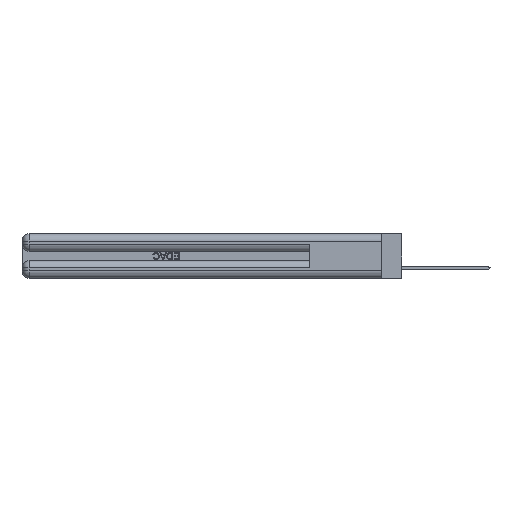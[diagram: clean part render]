
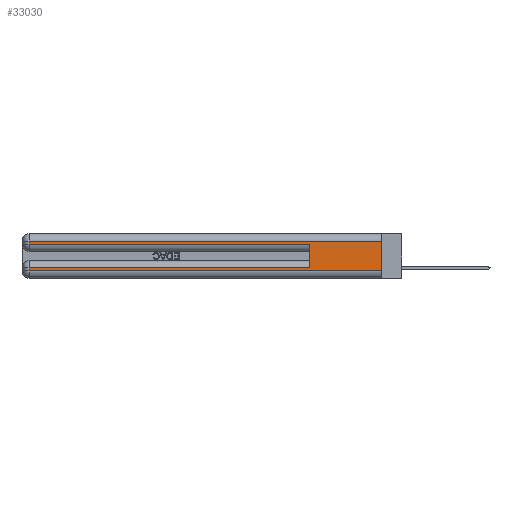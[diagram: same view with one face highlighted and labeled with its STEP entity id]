
A CAD part, left-side view. The second image highlights one B-rep face of the part: STEP entity #33030.
In plain terms, the highlighted planar face has unit normal (-1, 0, 0).
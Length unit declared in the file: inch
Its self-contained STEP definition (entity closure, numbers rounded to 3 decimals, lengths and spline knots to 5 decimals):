
#317 = VECTOR ( 'NONE', #15573, 39.37008 ) ;
#2219 = VECTOR ( 'NONE', #38193, 39.37008 ) ;
#2583 = CARTESIAN_POINT ( 'NONE',  ( 0., 0., 0.285 ) ) ;
#4704 = CARTESIAN_POINT ( 'NONE',  ( 0., 2.94, 0.31 ) ) ;
#5148 = ORIENTED_EDGE ( 'NONE', *, *, #36688, .F. ) ;
#5381 = ORIENTED_EDGE ( 'NONE', *, *, #43625, .T. ) ;
#7303 = AXIS2_PLACEMENT_3D ( 'NONE', #7928, #7403, #38817 ) ;
#7403 = DIRECTION ( 'NONE',  ( 1., 0., 0. ) ) ;
#7928 = CARTESIAN_POINT ( 'NONE',  ( 0., 0., 0.37 ) ) ;
#8430 = CARTESIAN_POINT ( 'NONE',  ( 0., 2.94, 0.06 ) ) ;
#8890 = VERTEX_POINT ( 'NONE', #9918 ) ;
#8986 = VECTOR ( 'NONE', #20823, 39.37008 ) ;
#9659 = CARTESIAN_POINT ( 'NONE',  ( 0., 0.6, 0.085 ) ) ;
#9918 = CARTESIAN_POINT ( 'NONE',  ( 0., 0., 0.31 ) ) ;
#10131 = EDGE_CURVE ( 'NONE', #13075, #24153, #19626, .T. ) ;
#10475 = DIRECTION ( 'NONE',  ( 0., 1., 0. ) ) ;
#11137 = PLANE ( 'NONE',  #7303 ) ;
#11789 = EDGE_LOOP ( 'NONE', ( #5148, #37324, #28812, #5381, #29724, #42980, #38608, #28479 ) ) ;
#11887 = EDGE_CURVE ( 'NONE', #49814, #44745, #32303, .T. ) ;
#12212 = CARTESIAN_POINT ( 'NONE',  ( 0., 0., 0.06 ) ) ;
#13075 = VERTEX_POINT ( 'NONE', #4704 ) ;
#13372 = DIRECTION ( 'NONE',  ( 0., 1., 0. ) ) ;
#13826 = FACE_OUTER_BOUND ( 'NONE', #11789, .T. ) ;
#14504 = EDGE_CURVE ( 'NONE', #49814, #30218, #38100, .T. ) ;
#14931 = EDGE_CURVE ( 'NONE', #44745, #48326, #49557, .T. ) ;
#15440 = VECTOR ( 'NONE', #34641, 39.37008 ) ;
#15573 = DIRECTION ( 'NONE',  ( 0., -1., 0. ) ) ;
#17324 = CARTESIAN_POINT ( 'NONE',  ( 0., 2.94, 0.37 ) ) ;
#19626 = LINE ( 'NONE', #35591, #43976 ) ;
#20183 = DIRECTION ( 'NONE',  ( 0., 0., -1. ) ) ;
#20823 = DIRECTION ( 'NONE',  ( 0., 0., -1. ) ) ;
#21083 = LINE ( 'NONE', #32241, #8986 ) ;
#22618 = EDGE_CURVE ( 'NONE', #8890, #13075, #23803, .T. ) ;
#23803 = LINE ( 'NONE', #29461, #44523 ) ;
#24153 = VERTEX_POINT ( 'NONE', #28552 ) ;
#24562 = LINE ( 'NONE', #2583, #15440 ) ;
#25000 = CARTESIAN_POINT ( 'NONE',  ( 0., 2.94, 0.085 ) ) ;
#25798 = LINE ( 'NONE', #12212, #317 ) ;
#28479 = ORIENTED_EDGE ( 'NONE', *, *, #43774, .T. ) ;
#28552 = CARTESIAN_POINT ( 'NONE',  ( 0., 2.94, 0.285 ) ) ;
#28812 = ORIENTED_EDGE ( 'NONE', *, *, #10131, .T. ) ;
#29461 = CARTESIAN_POINT ( 'NONE',  ( 0., 0., 0.31 ) ) ;
#29724 = ORIENTED_EDGE ( 'NONE', *, *, #14504, .F. ) ;
#30218 = VERTEX_POINT ( 'NONE', #48593 ) ;
#32241 = CARTESIAN_POINT ( 'NONE',  ( 0., 0., 0.37 ) ) ;
#32303 = LINE ( 'NONE', #44646, #44443 ) ;
#33030 = ADVANCED_FACE ( 'NONE', ( #13826 ), #11137, .F. ) ;
#34264 = CARTESIAN_POINT ( 'NONE',  ( 0., 0.6, 0.145 ) ) ;
#34641 = DIRECTION ( 'NONE',  ( 0., -1., 0. ) ) ;
#35591 = CARTESIAN_POINT ( 'NONE',  ( 0., 2.94, 0.37 ) ) ;
#36688 = EDGE_CURVE ( 'NONE', #8890, #45309, #21083, .T. ) ;
#37324 = ORIENTED_EDGE ( 'NONE', *, *, #22618, .T. ) ;
#38100 = LINE ( 'NONE', #34264, #2219 ) ;
#38193 = DIRECTION ( 'NONE',  ( 0., 0., 1. ) ) ;
#38608 = ORIENTED_EDGE ( 'NONE', *, *, #14931, .T. ) ;
#38817 = DIRECTION ( 'NONE',  ( 0., 0., -1. ) ) ;
#39518 = DIRECTION ( 'NONE',  ( 0., 0., -1. ) ) ;
#42523 = CARTESIAN_POINT ( 'NONE',  ( 0., 0., 0.06 ) ) ;
#42980 = ORIENTED_EDGE ( 'NONE', *, *, #11887, .T. ) ;
#43625 = EDGE_CURVE ( 'NONE', #24153, #30218, #24562, .T. ) ;
#43774 = EDGE_CURVE ( 'NONE', #48326, #45309, #25798, .T. ) ;
#43976 = VECTOR ( 'NONE', #39518, 39.37008 ) ;
#44443 = VECTOR ( 'NONE', #13372, 39.37008 ) ;
#44523 = VECTOR ( 'NONE', #10475, 39.37008 ) ;
#44646 = CARTESIAN_POINT ( 'NONE',  ( 0., 0., 0.085 ) ) ;
#44745 = VERTEX_POINT ( 'NONE', #25000 ) ;
#45306 = VECTOR ( 'NONE', #20183, 39.37008 ) ;
#45309 = VERTEX_POINT ( 'NONE', #42523 ) ;
#48326 = VERTEX_POINT ( 'NONE', #8430 ) ;
#48593 = CARTESIAN_POINT ( 'NONE',  ( 0., 0.6, 0.285 ) ) ;
#49557 = LINE ( 'NONE', #17324, #45306 ) ;
#49814 = VERTEX_POINT ( 'NONE', #9659 ) ;
